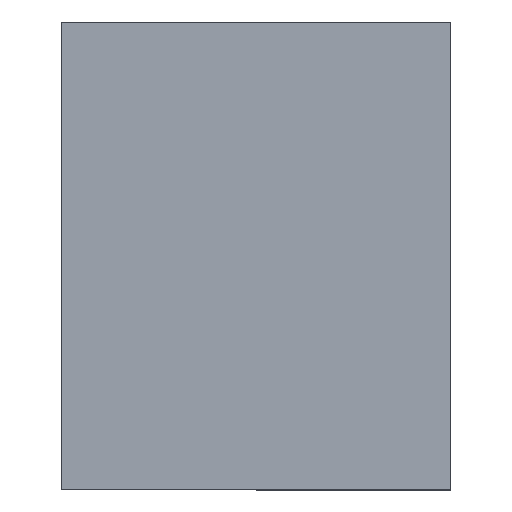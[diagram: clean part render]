
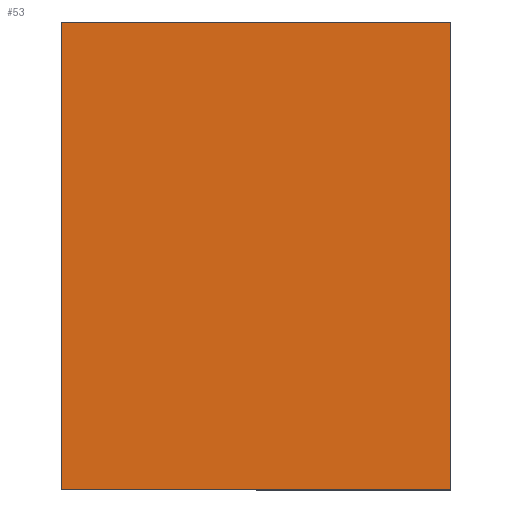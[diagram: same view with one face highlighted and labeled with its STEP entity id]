
A CAD part, top view. The second image highlights one B-rep face of the part: STEP entity #53.
In plain terms, the highlighted planar face has unit normal (0, 0, 1).
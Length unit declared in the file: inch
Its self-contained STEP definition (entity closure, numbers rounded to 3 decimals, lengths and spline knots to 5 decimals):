
#5 = VECTOR ( 'NONE', #170, 39.37008 ) ;
#7 = FACE_OUTER_BOUND ( 'NONE', #51, .T. ) ;
#9 = LINE ( 'NONE', #172, #5 ) ;
#13 = LINE ( 'NONE', #200, #114 ) ;
#26 = ORIENTED_EDGE ( 'NONE', *, *, #158, .T. ) ;
#27 = VECTOR ( 'NONE', #198, 39.37008 ) ;
#34 = VERTEX_POINT ( 'NONE', #175 ) ;
#37 = ORIENTED_EDGE ( 'NONE', *, *, #169, .T. ) ;
#39 = ORIENTED_EDGE ( 'NONE', *, *, #181, .T. ) ;
#46 = VERTEX_POINT ( 'NONE', #176 ) ;
#48 = LINE ( 'NONE', #81, #27 ) ;
#51 = EDGE_LOOP ( 'NONE', ( #39, #26, #37, #141 ) ) ;
#53 = ADVANCED_FACE ( 'NONE', ( #7 ), #155, .F. ) ;
#68 = LINE ( 'NONE', #177, #105 ) ;
#76 = VERTEX_POINT ( 'NONE', #126 ) ;
#81 = CARTESIAN_POINT ( 'NONE',  ( 0.99, -1.19, 0.1 ) ) ;
#105 = VECTOR ( 'NONE', #173, 39.37008 ) ;
#113 = AXIS2_PLACEMENT_3D ( 'NONE', #207, #145, #144 ) ;
#114 = VECTOR ( 'NONE', #182, 39.37008 ) ;
#126 = CARTESIAN_POINT ( 'NONE',  ( 0.99, 0., 0.1 ) ) ;
#141 = ORIENTED_EDGE ( 'NONE', *, *, #178, .T. ) ;
#144 = DIRECTION ( 'NONE',  ( -1., 0., 0. ) ) ;
#145 = DIRECTION ( 'NONE',  ( 0., 0., -1. ) ) ;
#155 = PLANE ( 'NONE',  #113 ) ;
#158 = EDGE_CURVE ( 'NONE', #34, #46, #48, .T. ) ;
#168 = VERTEX_POINT ( 'NONE', #190 ) ;
#169 = EDGE_CURVE ( 'NONE', #46, #76, #13, .T. ) ;
#170 = DIRECTION ( 'NONE',  ( 0., -1., 0. ) ) ;
#172 = CARTESIAN_POINT ( 'NONE',  ( 0., -1.19, 0.1 ) ) ;
#173 = DIRECTION ( 'NONE',  ( -1., 0., 0. ) ) ;
#175 = CARTESIAN_POINT ( 'NONE',  ( 0., -1.19, 0.1 ) ) ;
#176 = CARTESIAN_POINT ( 'NONE',  ( 0.99, -1.19, 0.1 ) ) ;
#177 = CARTESIAN_POINT ( 'NONE',  ( 0., 0., 0.1 ) ) ;
#178 = EDGE_CURVE ( 'NONE', #76, #168, #68, .T. ) ;
#181 = EDGE_CURVE ( 'NONE', #168, #34, #9, .T. ) ;
#182 = DIRECTION ( 'NONE',  ( 0., 1., 0. ) ) ;
#190 = CARTESIAN_POINT ( 'NONE',  ( 0., 0., 0.1 ) ) ;
#198 = DIRECTION ( 'NONE',  ( 1., 0., 0. ) ) ;
#200 = CARTESIAN_POINT ( 'NONE',  ( 0.99, 0., 0.1 ) ) ;
#207 = CARTESIAN_POINT ( 'NONE',  ( 0., 0., 0.1 ) ) ;
